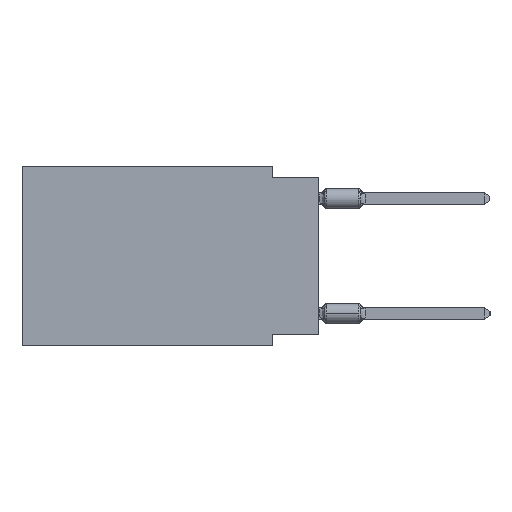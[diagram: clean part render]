
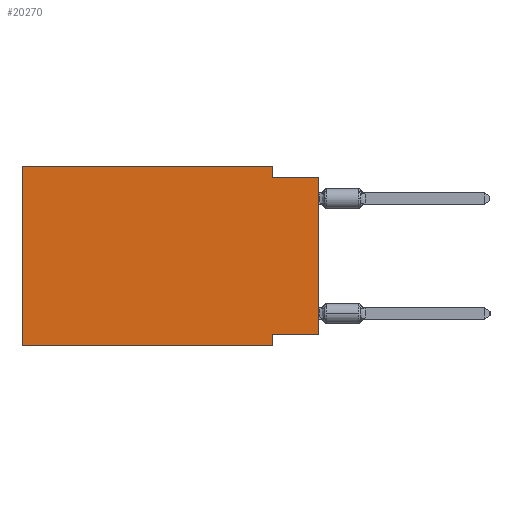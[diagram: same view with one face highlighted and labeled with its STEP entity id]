
A CAD part, left-side view. The second image highlights one B-rep face of the part: STEP entity #20270.
In plain terms, the highlighted planar face has unit normal (-1, 0, 0).
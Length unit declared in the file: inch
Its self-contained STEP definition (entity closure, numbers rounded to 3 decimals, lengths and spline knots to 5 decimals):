
#32 = VERTEX_POINT ( 'NONE', #21793 ) ;
#842 = VERTEX_POINT ( 'NONE', #22175 ) ;
#853 = EDGE_CURVE ( 'NONE', #18000, #12800, #11330, .T. ) ;
#1331 = LINE ( 'NONE', #16610, #9533 ) ;
#1473 = CARTESIAN_POINT ( 'NONE',  ( 0., 0.645, -0.39 ) ) ;
#1703 = LINE ( 'NONE', #4457, #19147 ) ;
#1964 = DIRECTION ( 'NONE',  ( 0., -1., 0. ) ) ;
#1988 = CARTESIAN_POINT ( 'NONE',  ( 0., 0., -0.365 ) ) ;
#2598 = EDGE_CURVE ( 'NONE', #21039, #21779, #18830, .T. ) ;
#3203 = CARTESIAN_POINT ( 'NONE',  ( 0., 0.645, 0. ) ) ;
#3477 = VECTOR ( 'NONE', #19588, 39.37008 ) ;
#4457 = CARTESIAN_POINT ( 'NONE',  ( 0., 0.645, 0. ) ) ;
#4576 = LINE ( 'NONE', #1988, #21134 ) ;
#4623 = CARTESIAN_POINT ( 'NONE',  ( 0., 0.1, -0.025 ) ) ;
#5036 = ORIENTED_EDGE ( 'NONE', *, *, #30133, .F. ) ;
#6141 = DIRECTION ( 'NONE',  ( 0., 0., 1. ) ) ;
#6628 = CARTESIAN_POINT ( 'NONE',  ( 0., 0.645, 0. ) ) ;
#7274 = LINE ( 'NONE', #1473, #20914 ) ;
#7878 = LINE ( 'NONE', #13542, #9698 ) ;
#8477 = ORIENTED_EDGE ( 'NONE', *, *, #13045, .T. ) ;
#9057 = LINE ( 'NONE', #14039, #32047 ) ;
#9533 = VECTOR ( 'NONE', #6141, 39.37008 ) ;
#9536 = CARTESIAN_POINT ( 'NONE',  ( 0., 0., -0.025 ) ) ;
#9698 = VECTOR ( 'NONE', #19043, 39.37008 ) ;
#10019 = VERTEX_POINT ( 'NONE', #18216 ) ;
#10629 = EDGE_LOOP ( 'NONE', ( #8477, #17787, #16341, #11522, #30264, #26649, #5036, #26321 ) ) ;
#11330 = LINE ( 'NONE', #19764, #3477 ) ;
#11522 = ORIENTED_EDGE ( 'NONE', *, *, #18502, .F. ) ;
#11806 = PLANE ( 'NONE',  #31278 ) ;
#12002 = EDGE_CURVE ( 'NONE', #10019, #842, #4576, .T. ) ;
#12457 = DIRECTION ( 'NONE',  ( 0., 1., 0. ) ) ;
#12800 = VERTEX_POINT ( 'NONE', #4623 ) ;
#13045 = EDGE_CURVE ( 'NONE', #10019, #23851, #1331, .T. ) ;
#13542 = CARTESIAN_POINT ( 'NONE',  ( 0., 0., -0.025 ) ) ;
#14039 = CARTESIAN_POINT ( 'NONE',  ( 0., 0.1, -0.39 ) ) ;
#16341 = ORIENTED_EDGE ( 'NONE', *, *, #853, .F. ) ;
#16610 = CARTESIAN_POINT ( 'NONE',  ( 0., 0., 0. ) ) ;
#17045 = EDGE_CURVE ( 'NONE', #12800, #23851, #7878, .T. ) ;
#17787 = ORIENTED_EDGE ( 'NONE', *, *, #17045, .F. ) ;
#18000 = VERTEX_POINT ( 'NONE', #28068 ) ;
#18106 = VECTOR ( 'NONE', #29545, 39.37008 ) ;
#18216 = CARTESIAN_POINT ( 'NONE',  ( 0., 0., -0.365 ) ) ;
#18502 = EDGE_CURVE ( 'NONE', #21779, #18000, #1703, .T. ) ;
#18830 = LINE ( 'NONE', #3203, #18106 ) ;
#19043 = DIRECTION ( 'NONE',  ( 0., -1., 0. ) ) ;
#19147 = VECTOR ( 'NONE', #30303, 39.37008 ) ;
#19588 = DIRECTION ( 'NONE',  ( 0., 0., -1. ) ) ;
#19764 = CARTESIAN_POINT ( 'NONE',  ( 0., 0.1, 0. ) ) ;
#20270 = ADVANCED_FACE ( 'NONE', ( #30098 ), #11806, .F. ) ;
#20914 = VECTOR ( 'NONE', #1964, 39.37008 ) ;
#21039 = VERTEX_POINT ( 'NONE', #29844 ) ;
#21134 = VECTOR ( 'NONE', #12457, 39.37008 ) ;
#21779 = VERTEX_POINT ( 'NONE', #6628 ) ;
#21793 = CARTESIAN_POINT ( 'NONE',  ( 0., 0.1, -0.39 ) ) ;
#22142 = DIRECTION ( 'NONE',  ( 1., 0., 0. ) ) ;
#22175 = CARTESIAN_POINT ( 'NONE',  ( 0., 0.1, -0.365 ) ) ;
#22816 = CARTESIAN_POINT ( 'NONE',  ( 0., 0.645, 0. ) ) ;
#23851 = VERTEX_POINT ( 'NONE', #9536 ) ;
#25058 = DIRECTION ( 'NONE',  ( 0., 0., -1. ) ) ;
#25535 = EDGE_CURVE ( 'NONE', #21039, #32, #7274, .T. ) ;
#26321 = ORIENTED_EDGE ( 'NONE', *, *, #12002, .F. ) ;
#26649 = ORIENTED_EDGE ( 'NONE', *, *, #25535, .T. ) ;
#28068 = CARTESIAN_POINT ( 'NONE',  ( 0., 0.1, 0. ) ) ;
#29545 = DIRECTION ( 'NONE',  ( 0., 0., 1. ) ) ;
#29844 = CARTESIAN_POINT ( 'NONE',  ( 0., 0.645, -0.39 ) ) ;
#30098 = FACE_OUTER_BOUND ( 'NONE', #10629, .T. ) ;
#30133 = EDGE_CURVE ( 'NONE', #842, #32, #9057, .T. ) ;
#30264 = ORIENTED_EDGE ( 'NONE', *, *, #2598, .F. ) ;
#30303 = DIRECTION ( 'NONE',  ( 0., -1., 0. ) ) ;
#30429 = DIRECTION ( 'NONE',  ( 0., 0., -1. ) ) ;
#31278 = AXIS2_PLACEMENT_3D ( 'NONE', #22816, #22142, #25058 ) ;
#32047 = VECTOR ( 'NONE', #30429, 39.37008 ) ;
